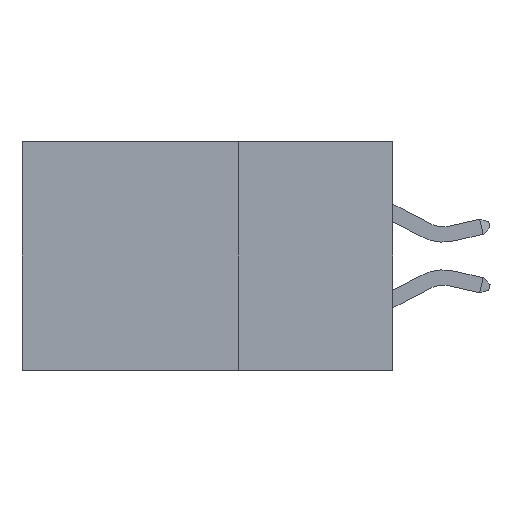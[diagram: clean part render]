
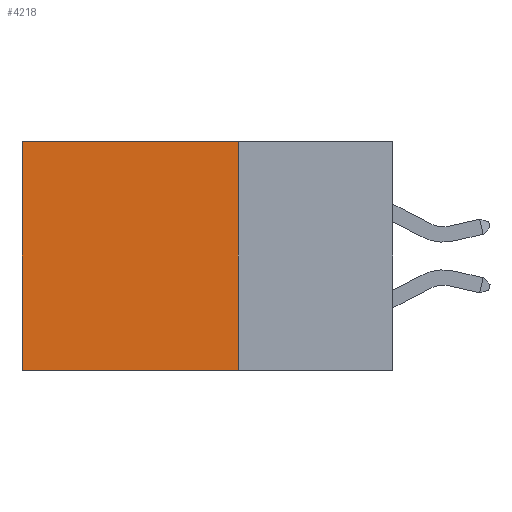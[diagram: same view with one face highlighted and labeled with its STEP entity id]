
A CAD part, left-side view. The second image highlights one B-rep face of the part: STEP entity #4218.
In plain terms, the highlighted planar face has unit normal (-1, 0, 0).
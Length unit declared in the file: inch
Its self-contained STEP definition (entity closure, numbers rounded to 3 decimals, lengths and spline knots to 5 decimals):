
#36 = DIRECTION ( 'NONE',  ( 0., 0., -1. ) ) ;
#345 = ORIENTED_EDGE ( 'NONE', *, *, #9350, .F. ) ;
#1153 = CARTESIAN_POINT ( 'NONE',  ( 0.2875, 0.25, 0. ) ) ;
#1256 = DIRECTION ( 'NONE',  ( 0., 0., -1. ) ) ;
#1698 = DIRECTION ( 'NONE',  ( 0., 1., 0. ) ) ;
#1750 = CARTESIAN_POINT ( 'NONE',  ( 0.2875, 0.25, -0.37 ) ) ;
#2177 = CARTESIAN_POINT ( 'NONE',  ( 0.2875, 0.6, -0.37 ) ) ;
#2227 = PLANE ( 'NONE',  #8924 ) ;
#2393 = LINE ( 'NONE', #1153, #9028 ) ;
#2733 = VECTOR ( 'NONE', #1256, 39.37008 ) ;
#3094 = VECTOR ( 'NONE', #9199, 39.37008 ) ;
#4180 = EDGE_CURVE ( 'NONE', #13041, #7086, #4210, .T. ) ;
#4210 = LINE ( 'NONE', #11382, #3094 ) ;
#4218 = ADVANCED_FACE ( 'NONE', ( #8838 ), #2227, .F. ) ;
#4423 = VECTOR ( 'NONE', #1698, 39.37008 ) ;
#4460 = VERTEX_POINT ( 'NONE', #14348 ) ;
#4743 = DIRECTION ( 'NONE',  ( 0., 1., 0. ) ) ;
#4808 = DIRECTION ( 'NONE',  ( 1., 0., 0. ) ) ;
#5870 = LINE ( 'NONE', #1750, #4423 ) ;
#5974 = CARTESIAN_POINT ( 'NONE',  ( 0.2875, 0.6, 0. ) ) ;
#6085 = CARTESIAN_POINT ( 'NONE',  ( 0.2875, 0.25, 0. ) ) ;
#7086 = VERTEX_POINT ( 'NONE', #2177 ) ;
#8000 = EDGE_LOOP ( 'NONE', ( #14441, #11613, #345, #9426 ) ) ;
#8436 = EDGE_CURVE ( 'NONE', #11698, #13041, #2393, .T. ) ;
#8838 = FACE_OUTER_BOUND ( 'NONE', #8000, .T. ) ;
#8924 = AXIS2_PLACEMENT_3D ( 'NONE', #13735, #4808, #36 ) ;
#9009 = EDGE_CURVE ( 'NONE', #4460, #7086, #5870, .T. ) ;
#9028 = VECTOR ( 'NONE', #4743, 39.37008 ) ;
#9199 = DIRECTION ( 'NONE',  ( 0., 0., -1. ) ) ;
#9350 = EDGE_CURVE ( 'NONE', #11698, #4460, #12974, .T. ) ;
#9426 = ORIENTED_EDGE ( 'NONE', *, *, #8436, .T. ) ;
#11382 = CARTESIAN_POINT ( 'NONE',  ( 0.2875, 0.6, 0. ) ) ;
#11613 = ORIENTED_EDGE ( 'NONE', *, *, #9009, .F. ) ;
#11698 = VERTEX_POINT ( 'NONE', #12723 ) ;
#12723 = CARTESIAN_POINT ( 'NONE',  ( 0.2875, 0.25, 0. ) ) ;
#12974 = LINE ( 'NONE', #6085, #2733 ) ;
#13041 = VERTEX_POINT ( 'NONE', #5974 ) ;
#13735 = CARTESIAN_POINT ( 'NONE',  ( 0.2875, 0.25, 0. ) ) ;
#14348 = CARTESIAN_POINT ( 'NONE',  ( 0.2875, 0.25, -0.37 ) ) ;
#14441 = ORIENTED_EDGE ( 'NONE', *, *, #4180, .T. ) ;
